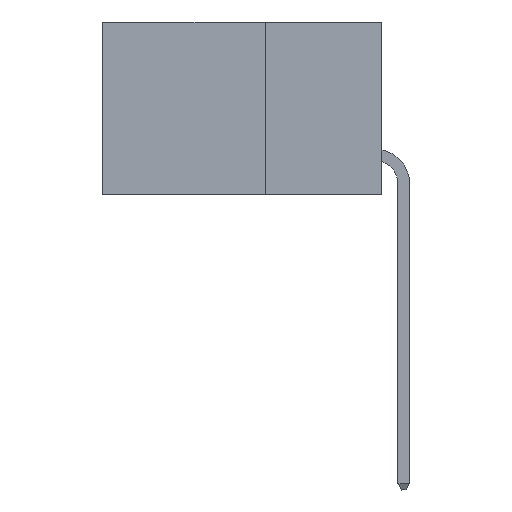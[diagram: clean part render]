
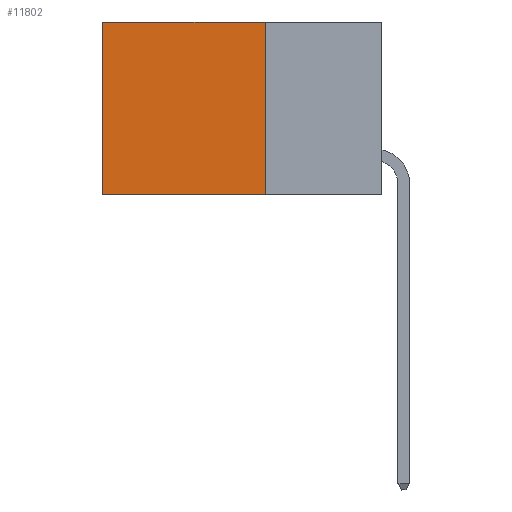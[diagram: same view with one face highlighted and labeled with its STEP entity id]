
A CAD part, left-side view. The second image highlights one B-rep face of the part: STEP entity #11802.
In plain terms, the highlighted planar face has unit normal (-1, 0, 0).
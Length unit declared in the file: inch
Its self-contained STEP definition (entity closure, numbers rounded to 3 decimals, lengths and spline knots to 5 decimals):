
#607 = EDGE_CURVE ( 'NONE', #24913, #22430, #5706, .T. ) ;
#1724 = ORIENTED_EDGE ( 'NONE', *, *, #607, .F. ) ;
#5706 = LINE ( 'NONE', #6753, #38941 ) ;
#5792 = DIRECTION ( 'NONE',  ( 1., 0., 0. ) ) ;
#6514 = CARTESIAN_POINT ( 'NONE',  ( 0.2875, 0.6, 0. ) ) ;
#6753 = CARTESIAN_POINT ( 'NONE',  ( 0.2875, 0.25, 0. ) ) ;
#7121 = EDGE_CURVE ( 'NONE', #24913, #35864, #45748, .T. ) ;
#9058 = DIRECTION ( 'NONE',  ( 0., 0., -1. ) ) ;
#9967 = DIRECTION ( 'NONE',  ( 0., 1., 0. ) ) ;
#10480 = VECTOR ( 'NONE', #35765, 39.37008 ) ;
#10840 = ORIENTED_EDGE ( 'NONE', *, *, #7121, .T. ) ;
#11802 = ADVANCED_FACE ( 'NONE', ( #33033 ), #23644, .F. ) ;
#17063 = VECTOR ( 'NONE', #9967, 39.37008 ) ;
#17557 = VECTOR ( 'NONE', #43588, 39.37008 ) ;
#18192 = LINE ( 'NONE', #34899, #17063 ) ;
#20281 = CARTESIAN_POINT ( 'NONE',  ( 0.2875, 0.25, -0.37 ) ) ;
#21007 = DIRECTION ( 'NONE',  ( 0., 0., -1. ) ) ;
#22430 = VERTEX_POINT ( 'NONE', #20281 ) ;
#23495 = EDGE_CURVE ( 'NONE', #35864, #31695, #35396, .T. ) ;
#23644 = PLANE ( 'NONE',  #39011 ) ;
#24064 = ORIENTED_EDGE ( 'NONE', *, *, #32843, .F. ) ;
#24620 = CARTESIAN_POINT ( 'NONE',  ( 0.2875, 0.6, 0. ) ) ;
#24913 = VERTEX_POINT ( 'NONE', #29868 ) ;
#26047 = EDGE_LOOP ( 'NONE', ( #34299, #24064, #1724, #10840 ) ) ;
#29868 = CARTESIAN_POINT ( 'NONE',  ( 0.2875, 0.25, 0. ) ) ;
#31695 = VERTEX_POINT ( 'NONE', #35129 ) ;
#32843 = EDGE_CURVE ( 'NONE', #22430, #31695, #18192, .T. ) ;
#33033 = FACE_OUTER_BOUND ( 'NONE', #26047, .T. ) ;
#34299 = ORIENTED_EDGE ( 'NONE', *, *, #23495, .T. ) ;
#34899 = CARTESIAN_POINT ( 'NONE',  ( 0.2875, 0.25, -0.37 ) ) ;
#35129 = CARTESIAN_POINT ( 'NONE',  ( 0.2875, 0.6, -0.37 ) ) ;
#35396 = LINE ( 'NONE', #6514, #10480 ) ;
#35765 = DIRECTION ( 'NONE',  ( 0., 0., -1. ) ) ;
#35864 = VERTEX_POINT ( 'NONE', #24620 ) ;
#38941 = VECTOR ( 'NONE', #21007, 39.37008 ) ;
#39011 = AXIS2_PLACEMENT_3D ( 'NONE', #40933, #5792, #9058 ) ;
#40933 = CARTESIAN_POINT ( 'NONE',  ( 0.2875, 0.25, 0. ) ) ;
#43588 = DIRECTION ( 'NONE',  ( 0., 1., 0. ) ) ;
#44363 = CARTESIAN_POINT ( 'NONE',  ( 0.2875, 0.25, 0. ) ) ;
#45748 = LINE ( 'NONE', #44363, #17557 ) ;
